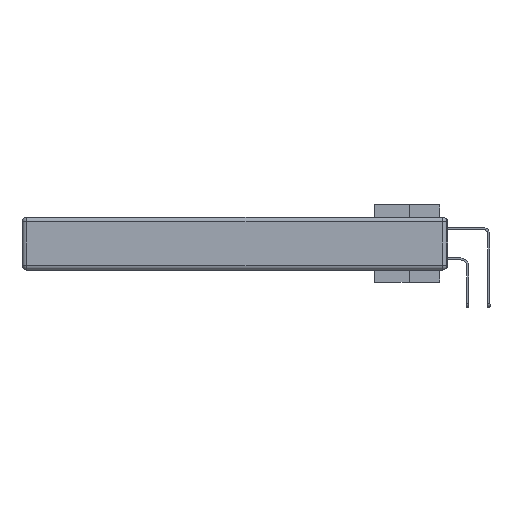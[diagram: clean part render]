
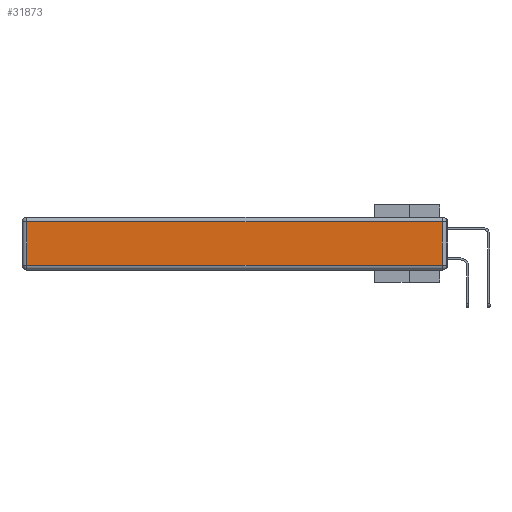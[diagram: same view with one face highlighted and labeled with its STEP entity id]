
A CAD part, left-side view. The second image highlights one B-rep face of the part: STEP entity #31873.
In plain terms, the highlighted planar face has unit normal (-1, 0, 0).
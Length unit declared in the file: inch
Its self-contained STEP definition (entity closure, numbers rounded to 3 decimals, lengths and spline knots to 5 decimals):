
#681 = EDGE_CURVE ( 'NONE', #26841, #17805, #19738, .T. ) ;
#4060 = AXIS2_PLACEMENT_3D ( 'NONE', #7974, #19230, #33755 ) ;
#4928 = CARTESIAN_POINT ( 'NONE',  ( 0., 2.72, -0.313 ) ) ;
#5107 = CARTESIAN_POINT ( 'NONE',  ( 0., 0.03, -0.03 ) ) ;
#5188 = VERTEX_POINT ( 'NONE', #7333 ) ;
#5733 = ORIENTED_EDGE ( 'NONE', *, *, #20050, .T. ) ;
#6330 = ORIENTED_EDGE ( 'NONE', *, *, #16907, .T. ) ;
#7333 = CARTESIAN_POINT ( 'NONE',  ( 0., 2.72, -0.03 ) ) ;
#7409 = DIRECTION ( 'NONE',  ( 0., 0., -1. ) ) ;
#7791 = CARTESIAN_POINT ( 'NONE',  ( 0., 2.72, -0.343 ) ) ;
#7974 = CARTESIAN_POINT ( 'NONE',  ( 0., 0., -0.343 ) ) ;
#8296 = DIRECTION ( 'NONE',  ( 0., 1., 0. ) ) ;
#10951 = CARTESIAN_POINT ( 'NONE',  ( 0., 0., -0.313 ) ) ;
#11497 = DIRECTION ( 'NONE',  ( 0., -1., 0. ) ) ;
#11501 = DIRECTION ( 'NONE',  ( 0., 0., 1. ) ) ;
#13297 = CARTESIAN_POINT ( 'NONE',  ( 0., 0.03, -0.313 ) ) ;
#15673 = LINE ( 'NONE', #7791, #21664 ) ;
#16115 = VECTOR ( 'NONE', #8296, 39.37008 ) ;
#16222 = ORIENTED_EDGE ( 'NONE', *, *, #26999, .T. ) ;
#16907 = EDGE_CURVE ( 'NONE', #27114, #5188, #36723, .T. ) ;
#17805 = VERTEX_POINT ( 'NONE', #13297 ) ;
#18252 = EDGE_LOOP ( 'NONE', ( #24717, #16222, #6330, #5733 ) ) ;
#19230 = DIRECTION ( 'NONE',  ( -1., 0., 0. ) ) ;
#19738 = LINE ( 'NONE', #10951, #21553 ) ;
#20050 = EDGE_CURVE ( 'NONE', #5188, #26841, #15673, .T. ) ;
#21553 = VECTOR ( 'NONE', #11497, 39.37008 ) ;
#21664 = VECTOR ( 'NONE', #7409, 39.37008 ) ;
#24717 = ORIENTED_EDGE ( 'NONE', *, *, #681, .T. ) ;
#26841 = VERTEX_POINT ( 'NONE', #4928 ) ;
#26999 = EDGE_CURVE ( 'NONE', #17805, #27114, #28692, .T. ) ;
#27114 = VERTEX_POINT ( 'NONE', #5107 ) ;
#28692 = LINE ( 'NONE', #36912, #30175 ) ;
#30175 = VECTOR ( 'NONE', #11501, 39.37008 ) ;
#31873 = ADVANCED_FACE ( 'NONE', ( #35826 ), #33391, .T. ) ;
#33391 = PLANE ( 'NONE',  #4060 ) ;
#33755 = DIRECTION ( 'NONE',  ( 0., 0., 1. ) ) ;
#33894 = CARTESIAN_POINT ( 'NONE',  ( 0., 2.75, -0.03 ) ) ;
#35826 = FACE_OUTER_BOUND ( 'NONE', #18252, .T. ) ;
#36723 = LINE ( 'NONE', #33894, #16115 ) ;
#36912 = CARTESIAN_POINT ( 'NONE',  ( 0., 0.03, -0.343 ) ) ;
